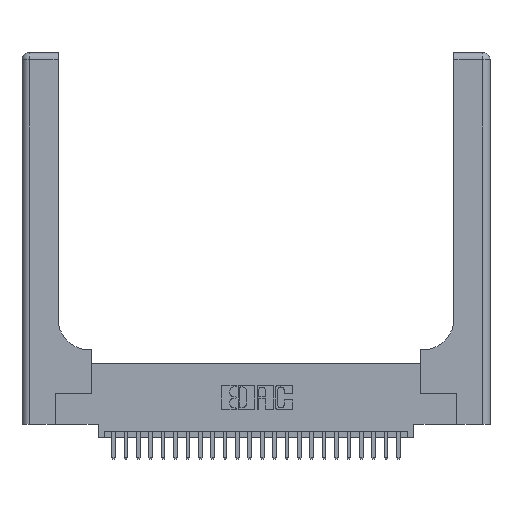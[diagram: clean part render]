
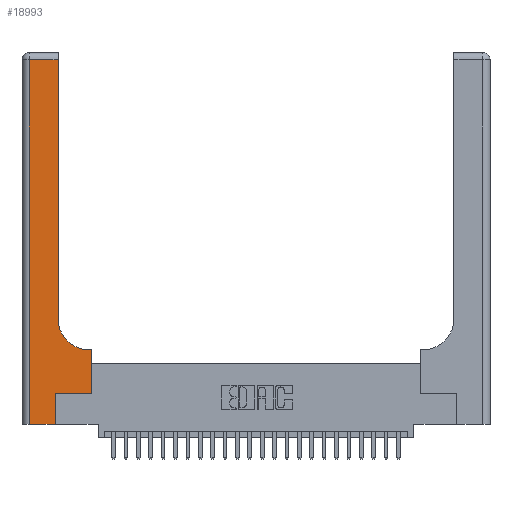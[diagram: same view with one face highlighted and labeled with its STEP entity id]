
A CAD part, top view. The second image highlights one B-rep face of the part: STEP entity #18993.
In plain terms, the highlighted planar face has unit normal (0, 0, 1).
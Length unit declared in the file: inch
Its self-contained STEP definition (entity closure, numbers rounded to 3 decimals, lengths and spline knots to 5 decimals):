
#672 = LINE ( 'NONE', #20879, #13217 ) ;
#803 = CIRCLE ( 'NONE', #25897, 0.25 ) ;
#1109 = LINE ( 'NONE', #4218, #22758 ) ;
#1334 = VECTOR ( 'NONE', #21702, 39.37008 ) ;
#2306 = CARTESIAN_POINT ( 'NONE',  ( 0.269, 0.25, 0.37 ) ) ;
#2340 = CARTESIAN_POINT ( 'NONE',  ( 0.2915, 0.85, 0.37 ) ) ;
#2694 = ORIENTED_EDGE ( 'NONE', *, *, #3167, .T. ) ;
#2827 = DIRECTION ( 'NONE',  ( 0., 1., 0. ) ) ;
#3089 = VECTOR ( 'NONE', #5597, 39.37008 ) ;
#3167 = EDGE_CURVE ( 'NONE', #19644, #4049, #5426, .T. ) ;
#3797 = VECTOR ( 'NONE', #8136, 39.37008 ) ;
#4049 = VERTEX_POINT ( 'NONE', #25292 ) ;
#4218 = CARTESIAN_POINT ( 'NONE',  ( 0.2915, 0.6, 0.37 ) ) ;
#5426 = LINE ( 'NONE', #22236, #3797 ) ;
#5597 = DIRECTION ( 'NONE',  ( -1., 0., 0. ) ) ;
#5852 = LINE ( 'NONE', #11749, #26468 ) ;
#6817 = LINE ( 'NONE', #17516, #1334 ) ;
#7033 = VERTEX_POINT ( 'NONE', #2340 ) ;
#7244 = VERTEX_POINT ( 'NONE', #10984 ) ;
#7545 = DIRECTION ( 'NONE',  ( 0., -1., 0. ) ) ;
#7647 = VERTEX_POINT ( 'NONE', #2306 ) ;
#8126 = ORIENTED_EDGE ( 'NONE', *, *, #24114, .T. ) ;
#8136 = DIRECTION ( 'NONE',  ( 1., 0., 0. ) ) ;
#8288 = DIRECTION ( 'NONE',  ( -1., 0., 0. ) ) ;
#8905 = CARTESIAN_POINT ( 'NONE',  ( 0.5585, 0.6, 0.37 ) ) ;
#9430 = DIRECTION ( 'NONE',  ( 1., 0., 0. ) ) ;
#9534 = ORIENTED_EDGE ( 'NONE', *, *, #18957, .T. ) ;
#9535 = CARTESIAN_POINT ( 'NONE',  ( 0.5415, 0.6, 0.37 ) ) ;
#9549 = LINE ( 'NONE', #19652, #3089 ) ;
#10984 = CARTESIAN_POINT ( 'NONE',  ( 0.5585, 0.25, 0.37 ) ) ;
#11128 = DIRECTION ( 'NONE',  ( 0., 0., -1. ) ) ;
#11213 = EDGE_CURVE ( 'NONE', #25016, #19644, #5852, .T. ) ;
#11380 = CARTESIAN_POINT ( 'NONE',  ( 0.2915, 2.94, 0.37 ) ) ;
#11749 = CARTESIAN_POINT ( 'NONE',  ( 0.06, 3., 0.37 ) ) ;
#12134 = DIRECTION ( 'NONE',  ( 1., 0., 0. ) ) ;
#12165 = VECTOR ( 'NONE', #2827, 39.37008 ) ;
#12240 = CARTESIAN_POINT ( 'NONE',  ( 0.06, 0., 0.37 ) ) ;
#12242 = ORIENTED_EDGE ( 'NONE', *, *, #24028, .T. ) ;
#12353 = AXIS2_PLACEMENT_3D ( 'NONE', #17348, #11128, #17258 ) ;
#13217 = VECTOR ( 'NONE', #14697, 39.37008 ) ;
#14035 = CARTESIAN_POINT ( 'NONE',  ( 0.06, 2.94, 0.37 ) ) ;
#14211 = EDGE_CURVE ( 'NONE', #18326, #14382, #1109, .T. ) ;
#14382 = VERTEX_POINT ( 'NONE', #9535 ) ;
#14697 = DIRECTION ( 'NONE',  ( 0., 1., 0. ) ) ;
#15514 = ORIENTED_EDGE ( 'NONE', *, *, #11213, .T. ) ;
#15738 = LINE ( 'NONE', #21438, #12165 ) ;
#17258 = DIRECTION ( 'NONE',  ( -1., 0., 0. ) ) ;
#17348 = CARTESIAN_POINT ( 'NONE',  ( 0., 3., 0.37 ) ) ;
#17354 = CARTESIAN_POINT ( 'NONE',  ( 0.5415, 0.85, 0.37 ) ) ;
#17516 = CARTESIAN_POINT ( 'NONE',  ( 0.2915, 3., 0.37 ) ) ;
#17667 = FACE_OUTER_BOUND ( 'NONE', #20751, .T. ) ;
#18326 = VERTEX_POINT ( 'NONE', #8905 ) ;
#18957 = EDGE_CURVE ( 'NONE', #4049, #7647, #15738, .T. ) ;
#18993 = ADVANCED_FACE ( 'NONE', ( #17667 ), #19531, .F. ) ;
#19515 = LINE ( 'NONE', #24530, #23411 ) ;
#19531 = PLANE ( 'NONE',  #12353 ) ;
#19644 = VERTEX_POINT ( 'NONE', #12240 ) ;
#19652 = CARTESIAN_POINT ( 'NONE',  ( 0., 2.94, 0.37 ) ) ;
#20109 = EDGE_CURVE ( 'NONE', #24132, #25016, #9549, .T. ) ;
#20751 = EDGE_LOOP ( 'NONE', ( #8126, #21477, #15514, #2694, #9534, #20788, #12242, #23900, #23321 ) ) ;
#20759 = EDGE_CURVE ( 'NONE', #7647, #7244, #19515, .T. ) ;
#20788 = ORIENTED_EDGE ( 'NONE', *, *, #20759, .T. ) ;
#20879 = CARTESIAN_POINT ( 'NONE',  ( 0.5585, 0.25, 0.37 ) ) ;
#20997 = EDGE_CURVE ( 'NONE', #14382, #7033, #803, .T. ) ;
#21438 = CARTESIAN_POINT ( 'NONE',  ( 0.269, 0., 0.37 ) ) ;
#21477 = ORIENTED_EDGE ( 'NONE', *, *, #20109, .T. ) ;
#21702 = DIRECTION ( 'NONE',  ( 0., 1., 0. ) ) ;
#22236 = CARTESIAN_POINT ( 'NONE',  ( 0., 0., 0.37 ) ) ;
#22758 = VECTOR ( 'NONE', #8288, 39.37008 ) ;
#23321 = ORIENTED_EDGE ( 'NONE', *, *, #20997, .T. ) ;
#23411 = VECTOR ( 'NONE', #12134, 39.37008 ) ;
#23900 = ORIENTED_EDGE ( 'NONE', *, *, #14211, .T. ) ;
#24028 = EDGE_CURVE ( 'NONE', #7244, #18326, #672, .T. ) ;
#24114 = EDGE_CURVE ( 'NONE', #7033, #24132, #6817, .T. ) ;
#24132 = VERTEX_POINT ( 'NONE', #11380 ) ;
#24530 = CARTESIAN_POINT ( 'NONE',  ( 0.269, 0.25, 0.37 ) ) ;
#25016 = VERTEX_POINT ( 'NONE', #14035 ) ;
#25292 = CARTESIAN_POINT ( 'NONE',  ( 0.269, 0., 0.37 ) ) ;
#25563 = DIRECTION ( 'NONE',  ( 0., 0., -1. ) ) ;
#25897 = AXIS2_PLACEMENT_3D ( 'NONE', #17354, #25563, #9430 ) ;
#26468 = VECTOR ( 'NONE', #7545, 39.37008 ) ;
